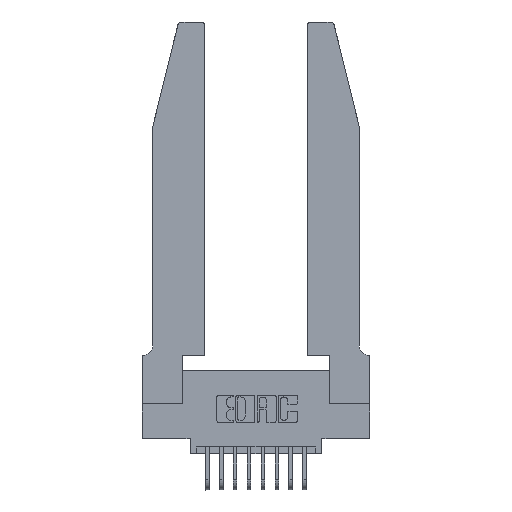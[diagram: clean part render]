
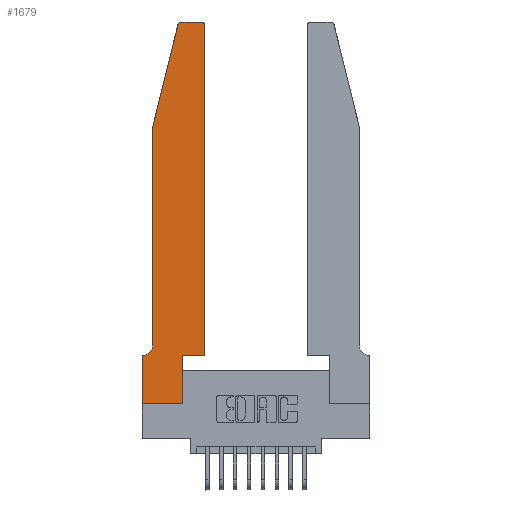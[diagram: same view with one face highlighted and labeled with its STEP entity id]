
A CAD part, top view. The second image highlights one B-rep face of the part: STEP entity #1679.
In plain terms, the highlighted planar face has unit normal (0, 0, 1).
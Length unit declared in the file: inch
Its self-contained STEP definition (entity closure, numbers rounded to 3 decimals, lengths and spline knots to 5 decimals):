
#189 = CARTESIAN_POINT ( 'NONE',  ( 0.4505, 2.72, 0.37 ) ) ;
#695 = DIRECTION ( 'NONE',  ( -1., 0., 0. ) ) ;
#701 = CARTESIAN_POINT ( 'NONE',  ( 0.2865, 0.35, 0.37 ) ) ;
#780 = CARTESIAN_POINT ( 'NONE',  ( 0.25487, 2.72718, 0.37 ) ) ;
#1093 = CARTESIAN_POINT ( 'NONE',  ( 0., 0.35, 0.37 ) ) ;
#1187 = VERTEX_POINT ( 'NONE', #12650 ) ;
#1230 = VERTEX_POINT ( 'NONE', #12486 ) ;
#1413 = CARTESIAN_POINT ( 'NONE',  ( 0.4505, 0.35, 0.37 ) ) ;
#1423 = ORIENTED_EDGE ( 'NONE', *, *, #13865, .T. ) ;
#1489 = DIRECTION ( 'NONE',  ( 1., 0., 0. ) ) ;
#1633 = VERTEX_POINT ( 'NONE', #9950 ) ;
#1679 = ADVANCED_FACE ( 'NONE', ( #10906 ), #2903, .T. ) ;
#1723 = VECTOR ( 'NONE', #10950, 39.37008 ) ;
#1776 = EDGE_CURVE ( 'NONE', #2381, #4179, #3297, .T. ) ;
#1892 = DIRECTION ( 'NONE',  ( 0., 1., 0. ) ) ;
#1963 = ORIENTED_EDGE ( 'NONE', *, *, #5531, .T. ) ;
#1966 = AXIS2_PLACEMENT_3D ( 'NONE', #15123, #7957, #695 ) ;
#2117 = CARTESIAN_POINT ( 'NONE',  ( 0., 0., 0.37 ) ) ;
#2366 = VECTOR ( 'NONE', #8651, 39.37008 ) ;
#2381 = VERTEX_POINT ( 'NONE', #5477 ) ;
#2393 = AXIS2_PLACEMENT_3D ( 'NONE', #3624, #12114, #4853 ) ;
#2439 = VECTOR ( 'NONE', #9458, 39.37008 ) ;
#2609 = CARTESIAN_POINT ( 'NONE',  ( 0.0755, 0.35, 0.37 ) ) ;
#2625 = VERTEX_POINT ( 'NONE', #1093 ) ;
#2728 = DIRECTION ( 'NONE',  ( -1., 0., 0. ) ) ;
#2812 = EDGE_CURVE ( 'NONE', #5571, #2625, #15192, .T. ) ;
#2861 = EDGE_CURVE ( 'NONE', #4179, #3334, #14436, .T. ) ;
#2903 = PLANE ( 'NONE',  #12969 ) ;
#3297 = LINE ( 'NONE', #701, #12585 ) ;
#3334 = VERTEX_POINT ( 'NONE', #1413 ) ;
#3573 = EDGE_CURVE ( 'NONE', #13248, #5571, #11796, .T. ) ;
#3624 = CARTESIAN_POINT ( 'NONE',  ( 0.4205, 2.72, 0.37 ) ) ;
#3986 = VECTOR ( 'NONE', #8531, 39.37008 ) ;
#4083 = VERTEX_POINT ( 'NONE', #780 ) ;
#4099 = DIRECTION ( 'NONE',  ( 0., 0., 1. ) ) ;
#4179 = VERTEX_POINT ( 'NONE', #14213 ) ;
#4481 = CIRCLE ( 'NONE', #5092, 0.03 ) ;
#4574 = DIRECTION ( 'NONE',  ( -0.239, -0.971, 0. ) ) ;
#4634 = CARTESIAN_POINT ( 'NONE',  ( 0.0055, 0.35, 0.37 ) ) ;
#4835 = LINE ( 'NONE', #11188, #14467 ) ;
#4853 = DIRECTION ( 'NONE',  ( 1., 0., 0. ) ) ;
#4915 = LINE ( 'NONE', #9728, #1723 ) ;
#5020 = EDGE_CURVE ( 'NONE', #8311, #11477, #11754, .T. ) ;
#5092 = AXIS2_PLACEMENT_3D ( 'NONE', #6716, #15090, #7930 ) ;
#5211 = ORIENTED_EDGE ( 'NONE', *, *, #12847, .T. ) ;
#5456 = LINE ( 'NONE', #2117, #15055 ) ;
#5477 = CARTESIAN_POINT ( 'NONE',  ( 0.2865, 0., 0.37 ) ) ;
#5531 = EDGE_CURVE ( 'NONE', #4083, #1230, #12122, .T. ) ;
#5571 = VERTEX_POINT ( 'NONE', #4634 ) ;
#6716 = CARTESIAN_POINT ( 'NONE',  ( 0.284, 2.72, 0.37 ) ) ;
#6825 = ORIENTED_EDGE ( 'NONE', *, *, #5020, .T. ) ;
#7268 = LINE ( 'NONE', #9693, #3986 ) ;
#7930 = DIRECTION ( 'NONE',  ( 1., 0., 0. ) ) ;
#7957 = DIRECTION ( 'NONE',  ( 0., 0., -1. ) ) ;
#8234 = CARTESIAN_POINT ( 'NONE',  ( 0.0755, 2., 0.37 ) ) ;
#8311 = VERTEX_POINT ( 'NONE', #189 ) ;
#8337 = CARTESIAN_POINT ( 'NONE',  ( 0.4205, 2.75, 0.37 ) ) ;
#8531 = DIRECTION ( 'NONE',  ( 0., 1., 0. ) ) ;
#8541 = VECTOR ( 'NONE', #4574, 39.37008 ) ;
#8651 = DIRECTION ( 'NONE',  ( -1., 0., 0. ) ) ;
#8692 = EDGE_CURVE ( 'NONE', #3334, #8311, #7268, .T. ) ;
#8972 = ORIENTED_EDGE ( 'NONE', *, *, #3573, .T. ) ;
#9001 = ORIENTED_EDGE ( 'NONE', *, *, #2812, .T. ) ;
#9305 = EDGE_CURVE ( 'NONE', #1633, #2381, #4915, .T. ) ;
#9458 = DIRECTION ( 'NONE',  ( 0., -1., 0. ) ) ;
#9514 = CARTESIAN_POINT ( 'NONE',  ( 0.0755, 0.42, 0.37 ) ) ;
#9637 = ORIENTED_EDGE ( 'NONE', *, *, #11415, .T. ) ;
#9693 = CARTESIAN_POINT ( 'NONE',  ( 0.4505, 0.35, 0.37 ) ) ;
#9728 = CARTESIAN_POINT ( 'NONE',  ( 0., 0., 0.37 ) ) ;
#9899 = ORIENTED_EDGE ( 'NONE', *, *, #2861, .T. ) ;
#9950 = CARTESIAN_POINT ( 'NONE',  ( 0., 0., 0.37 ) ) ;
#10590 = DIRECTION ( 'NONE',  ( 0., -1., 0. ) ) ;
#10637 = CARTESIAN_POINT ( 'NONE',  ( 0.0755, 2., 0.37 ) ) ;
#10666 = ORIENTED_EDGE ( 'NONE', *, *, #8692, .T. ) ;
#10906 = FACE_OUTER_BOUND ( 'NONE', #13488, .T. ) ;
#10950 = DIRECTION ( 'NONE',  ( 1., 0., 0. ) ) ;
#11188 = CARTESIAN_POINT ( 'NONE',  ( 0.2605, 2.75, 0.37 ) ) ;
#11370 = CARTESIAN_POINT ( 'NONE',  ( 0., 0.35, 0.37 ) ) ;
#11415 = EDGE_CURVE ( 'NONE', #1230, #13248, #12093, .T. ) ;
#11477 = VERTEX_POINT ( 'NONE', #8337 ) ;
#11754 = CIRCLE ( 'NONE', #2393, 0.03 ) ;
#11796 = CIRCLE ( 'NONE', #1966, 0.07 ) ;
#12093 = LINE ( 'NONE', #8234, #2439 ) ;
#12114 = DIRECTION ( 'NONE',  ( 0., 0., 1. ) ) ;
#12122 = LINE ( 'NONE', #10637, #8541 ) ;
#12333 = CARTESIAN_POINT ( 'NONE',  ( 0.4505, 0.35, 0.37 ) ) ;
#12486 = CARTESIAN_POINT ( 'NONE',  ( 0.0755, 2., 0.37 ) ) ;
#12580 = DIRECTION ( 'NONE',  ( 1., 0., 0. ) ) ;
#12585 = VECTOR ( 'NONE', #1892, 39.37008 ) ;
#12650 = CARTESIAN_POINT ( 'NONE',  ( 0.284, 2.75, 0.37 ) ) ;
#12775 = ORIENTED_EDGE ( 'NONE', *, *, #1776, .T. ) ;
#12847 = EDGE_CURVE ( 'NONE', #11477, #1187, #4835, .T. ) ;
#12969 = AXIS2_PLACEMENT_3D ( 'NONE', #11370, #4099, #12580 ) ;
#13248 = VERTEX_POINT ( 'NONE', #9514 ) ;
#13427 = ORIENTED_EDGE ( 'NONE', *, *, #9305, .T. ) ;
#13488 = EDGE_LOOP ( 'NONE', ( #5211, #13808, #1963, #9637, #8972, #9001, #1423, #13427, #12775, #9899, #10666, #6825 ) ) ;
#13703 = EDGE_CURVE ( 'NONE', #1187, #4083, #4481, .T. ) ;
#13808 = ORIENTED_EDGE ( 'NONE', *, *, #13703, .T. ) ;
#13865 = EDGE_CURVE ( 'NONE', #2625, #1633, #5456, .T. ) ;
#14213 = CARTESIAN_POINT ( 'NONE',  ( 0.2865, 0.35, 0.37 ) ) ;
#14436 = LINE ( 'NONE', #12333, #14814 ) ;
#14467 = VECTOR ( 'NONE', #2728, 39.37008 ) ;
#14814 = VECTOR ( 'NONE', #1489, 39.37008 ) ;
#15055 = VECTOR ( 'NONE', #10590, 39.37008 ) ;
#15090 = DIRECTION ( 'NONE',  ( 0., 0., 1. ) ) ;
#15123 = CARTESIAN_POINT ( 'NONE',  ( 0.0055, 0.42, 0.37 ) ) ;
#15192 = LINE ( 'NONE', #2609, #2366 ) ;
